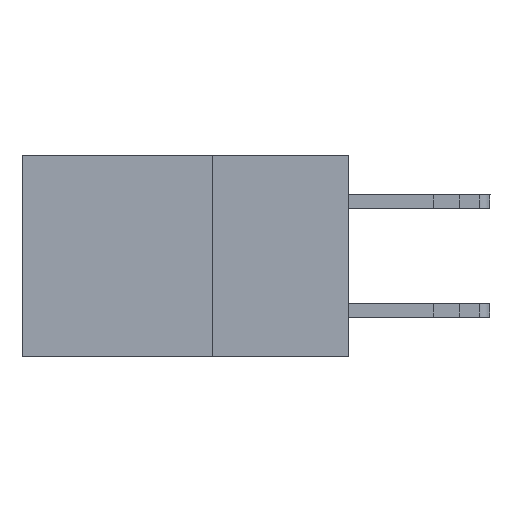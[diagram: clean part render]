
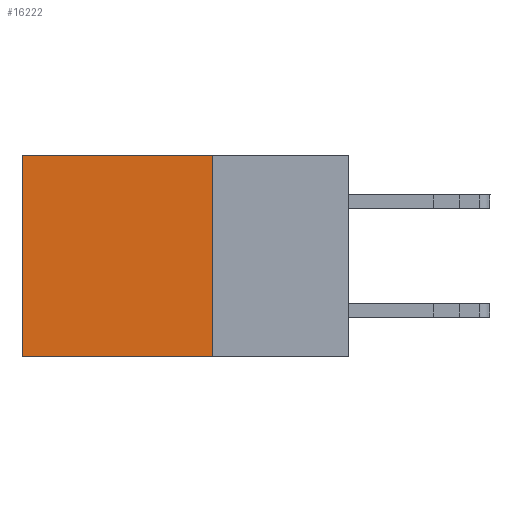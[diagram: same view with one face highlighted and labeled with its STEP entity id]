
A CAD part, left-side view. The second image highlights one B-rep face of the part: STEP entity #16222.
In plain terms, the highlighted planar face has unit normal (-1, 0, 0).
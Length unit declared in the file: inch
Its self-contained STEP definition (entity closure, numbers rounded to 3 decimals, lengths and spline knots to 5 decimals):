
#188 = CARTESIAN_POINT ( 'NONE',  ( 0.298, 0.6, 0. ) ) ;
#521 = LINE ( 'NONE', #8413, #11240 ) ;
#1003 = VECTOR ( 'NONE', #9945, 39.37008 ) ;
#1402 = EDGE_LOOP ( 'NONE', ( #10121, #10383, #13378, #4754 ) ) ;
#2014 = VERTEX_POINT ( 'NONE', #188 ) ;
#2097 = CARTESIAN_POINT ( 'NONE',  ( 0.298, 0.6, -0.37 ) ) ;
#2227 = VECTOR ( 'NONE', #2323, 39.37008 ) ;
#2323 = DIRECTION ( 'NONE',  ( 0., 0., -1. ) ) ;
#2358 = CARTESIAN_POINT ( 'NONE',  ( 0.298, 0.25, 0. ) ) ;
#3583 = FACE_OUTER_BOUND ( 'NONE', #1402, .T. ) ;
#4704 = CARTESIAN_POINT ( 'NONE',  ( 0.298, 0.25, -0.37 ) ) ;
#4754 = ORIENTED_EDGE ( 'NONE', *, *, #5467, .T. ) ;
#4768 = DIRECTION ( 'NONE',  ( 1., 0., 0. ) ) ;
#5467 = EDGE_CURVE ( 'NONE', #15221, #2014, #8299, .T. ) ;
#8299 = LINE ( 'NONE', #11956, #15325 ) ;
#8413 = CARTESIAN_POINT ( 'NONE',  ( 0.298, 0.6, 0. ) ) ;
#9945 = DIRECTION ( 'NONE',  ( 0., 1., 0. ) ) ;
#10011 = PLANE ( 'NONE',  #14667 ) ;
#10121 = ORIENTED_EDGE ( 'NONE', *, *, #12011, .T. ) ;
#10383 = ORIENTED_EDGE ( 'NONE', *, *, #15690, .F. ) ;
#10629 = CARTESIAN_POINT ( 'NONE',  ( 0.298, 0.25, -0.37 ) ) ;
#11240 = VECTOR ( 'NONE', #13821, 39.37008 ) ;
#11956 = CARTESIAN_POINT ( 'NONE',  ( 0.298, 0.25, 0. ) ) ;
#12011 = EDGE_CURVE ( 'NONE', #2014, #13058, #521, .T. ) ;
#12370 = CARTESIAN_POINT ( 'NONE',  ( 0.298, 0.25, 0. ) ) ;
#12551 = LINE ( 'NONE', #14097, #2227 ) ;
#12743 = DIRECTION ( 'NONE',  ( 0., 1., 0. ) ) ;
#13058 = VERTEX_POINT ( 'NONE', #2097 ) ;
#13378 = ORIENTED_EDGE ( 'NONE', *, *, #13449, .F. ) ;
#13449 = EDGE_CURVE ( 'NONE', #15221, #15444, #12551, .T. ) ;
#13821 = DIRECTION ( 'NONE',  ( 0., 0., -1. ) ) ;
#14097 = CARTESIAN_POINT ( 'NONE',  ( 0.298, 0.25, 0. ) ) ;
#14667 = AXIS2_PLACEMENT_3D ( 'NONE', #2358, #4768, #15235 ) ;
#15221 = VERTEX_POINT ( 'NONE', #12370 ) ;
#15235 = DIRECTION ( 'NONE',  ( 0., 0., -1. ) ) ;
#15325 = VECTOR ( 'NONE', #12743, 39.37008 ) ;
#15444 = VERTEX_POINT ( 'NONE', #10629 ) ;
#15690 = EDGE_CURVE ( 'NONE', #15444, #13058, #16455, .T. ) ;
#16222 = ADVANCED_FACE ( 'NONE', ( #3583 ), #10011, .F. ) ;
#16455 = LINE ( 'NONE', #4704, #1003 ) ;
